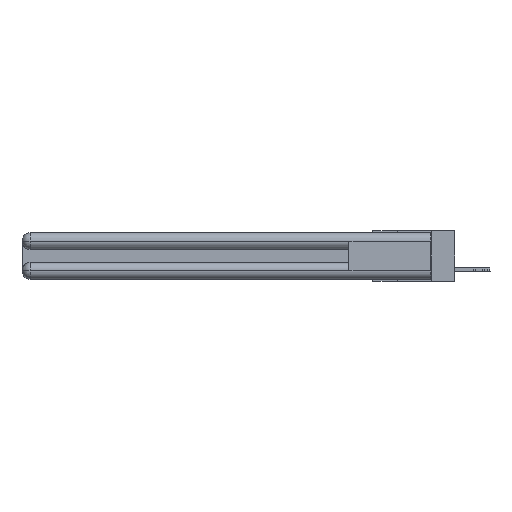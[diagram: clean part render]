
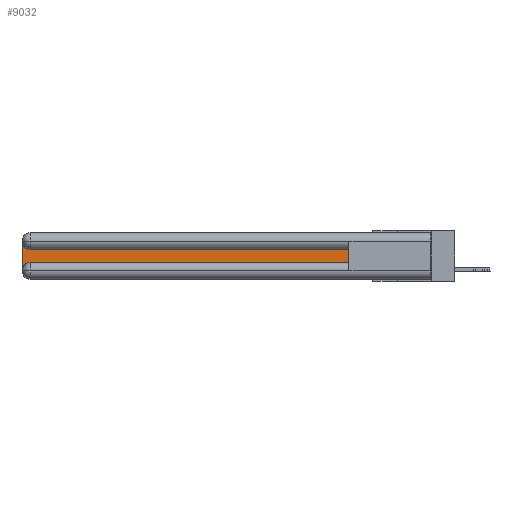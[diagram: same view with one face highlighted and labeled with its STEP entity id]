
A CAD part, left-side view. The second image highlights one B-rep face of the part: STEP entity #9032.
In plain terms, the highlighted planar face has unit normal (-1, 0, 0).
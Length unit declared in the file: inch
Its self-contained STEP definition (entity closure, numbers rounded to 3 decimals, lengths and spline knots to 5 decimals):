
#230 = VECTOR ( 'NONE', #20430, 39.37008 ) ;
#2221 = CIRCLE ( 'NONE', #23973, 0.06 ) ;
#3643 = CARTESIAN_POINT ( 'NONE',  ( 0.075, 0.6, -0.1225 ) ) ;
#4388 = ORIENTED_EDGE ( 'NONE', *, *, #15276, .T. ) ;
#5294 = EDGE_CURVE ( 'NONE', #7320, #25314, #16995, .T. ) ;
#5421 = CARTESIAN_POINT ( 'NONE',  ( 0.075, 3., -0.2175 ) ) ;
#6677 = ORIENTED_EDGE ( 'NONE', *, *, #5294, .T. ) ;
#6798 = CARTESIAN_POINT ( 'NONE',  ( 0.075, 2.94, -0.2775 ) ) ;
#6908 = DIRECTION ( 'NONE',  ( 0., 0., -1. ) ) ;
#7243 = LINE ( 'NONE', #13139, #11170 ) ;
#7320 = VERTEX_POINT ( 'NONE', #20712 ) ;
#8463 = CARTESIAN_POINT ( 'NONE',  ( 0.075, 0.6, -0.2175 ) ) ;
#8474 = EDGE_CURVE ( 'NONE', #23671, #31423, #2221, .T. ) ;
#8532 = FACE_OUTER_BOUND ( 'NONE', #18442, .T. ) ;
#8959 = VECTOR ( 'NONE', #25099, 39.37008 ) ;
#9032 = ADVANCED_FACE ( 'NONE', ( #8532 ), #26420, .F. ) ;
#10513 = LINE ( 'NONE', #5421, #230 ) ;
#10665 = EDGE_CURVE ( 'NONE', #15921, #23671, #7243, .T. ) ;
#11170 = VECTOR ( 'NONE', #13353, 39.37008 ) ;
#11334 = CARTESIAN_POINT ( 'NONE',  ( 0.075, 3., -0.1225 ) ) ;
#12098 = DIRECTION ( 'NONE',  ( 1., 0., 0. ) ) ;
#12883 = CARTESIAN_POINT ( 'NONE',  ( 0.075, 0.6, -0.2175 ) ) ;
#13139 = CARTESIAN_POINT ( 'NONE',  ( 0.075, 0.6, -0.1225 ) ) ;
#13353 = DIRECTION ( 'NONE',  ( 0., 1., 0. ) ) ;
#13857 = DIRECTION ( 'NONE',  ( 0., 0., -1. ) ) ;
#14591 = ORIENTED_EDGE ( 'NONE', *, *, #10665, .T. ) ;
#14835 = CARTESIAN_POINT ( 'NONE',  ( 0.075, 3., -0.0625 ) ) ;
#15276 = EDGE_CURVE ( 'NONE', #31423, #7320, #10513, .T. ) ;
#15921 = VERTEX_POINT ( 'NONE', #3643 ) ;
#15988 = ORIENTED_EDGE ( 'NONE', *, *, #18164, .T. ) ;
#16995 = CIRCLE ( 'NONE', #31168, 0.06 ) ;
#17431 = ORIENTED_EDGE ( 'NONE', *, *, #32141, .T. ) ;
#18164 = EDGE_CURVE ( 'NONE', #25314, #32495, #18178, .T. ) ;
#18178 = LINE ( 'NONE', #18746, #24857 ) ;
#18442 = EDGE_LOOP ( 'NONE', ( #14591, #32658, #4388, #6677, #15988, #17431 ) ) ;
#18746 = CARTESIAN_POINT ( 'NONE',  ( 0.075, 0.6, -0.2175 ) ) ;
#18868 = CARTESIAN_POINT ( 'NONE',  ( 0.075, 2.94, -0.1225 ) ) ;
#19714 = CARTESIAN_POINT ( 'NONE',  ( 0.075, 2.94, -0.0625 ) ) ;
#20144 = DIRECTION ( 'NONE',  ( 0., 0., -1. ) ) ;
#20430 = DIRECTION ( 'NONE',  ( 0., 0., -1. ) ) ;
#20712 = CARTESIAN_POINT ( 'NONE',  ( 0.075, 3., -0.2775 ) ) ;
#21043 = AXIS2_PLACEMENT_3D ( 'NONE', #11334, #28962, #13857 ) ;
#22349 = LINE ( 'NONE', #12883, #8959 ) ;
#23671 = VERTEX_POINT ( 'NONE', #18868 ) ;
#23973 = AXIS2_PLACEMENT_3D ( 'NONE', #19714, #32292, #20144 ) ;
#24857 = VECTOR ( 'NONE', #29219, 39.37008 ) ;
#25099 = DIRECTION ( 'NONE',  ( 0., 0., 1. ) ) ;
#25183 = CARTESIAN_POINT ( 'NONE',  ( 0.075, 2.94, -0.2175 ) ) ;
#25314 = VERTEX_POINT ( 'NONE', #25183 ) ;
#26420 = PLANE ( 'NONE',  #21043 ) ;
#28962 = DIRECTION ( 'NONE',  ( 1., 0., 0. ) ) ;
#29219 = DIRECTION ( 'NONE',  ( 0., -1., 0. ) ) ;
#31168 = AXIS2_PLACEMENT_3D ( 'NONE', #6798, #12098, #6908 ) ;
#31423 = VERTEX_POINT ( 'NONE', #14835 ) ;
#32141 = EDGE_CURVE ( 'NONE', #32495, #15921, #22349, .T. ) ;
#32292 = DIRECTION ( 'NONE',  ( 1., 0., 0. ) ) ;
#32495 = VERTEX_POINT ( 'NONE', #8463 ) ;
#32658 = ORIENTED_EDGE ( 'NONE', *, *, #8474, .T. ) ;
